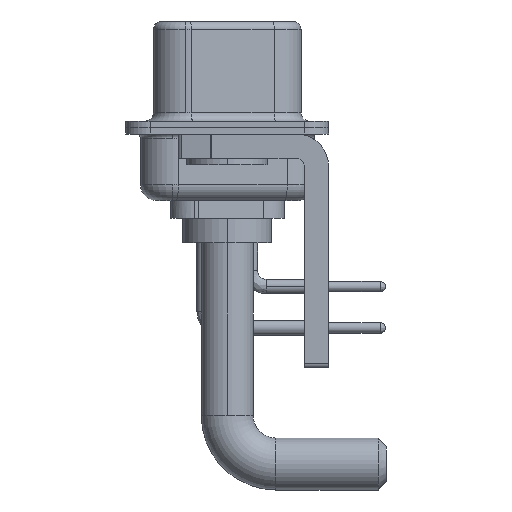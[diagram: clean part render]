
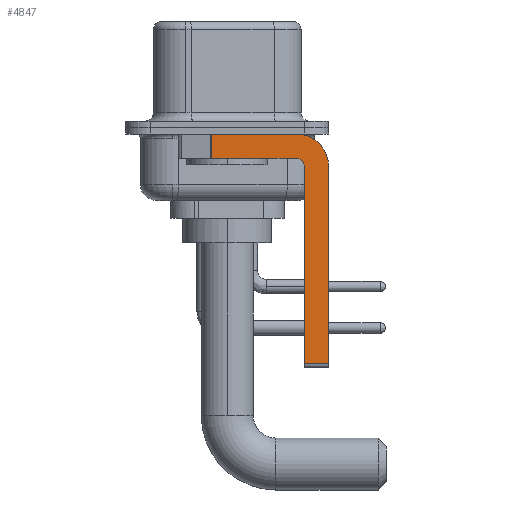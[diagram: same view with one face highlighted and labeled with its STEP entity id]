
A CAD part, left-side view. The second image highlights one B-rep face of the part: STEP entity #4847.
In plain terms, the highlighted planar face has unit normal (-1, 0, 0).
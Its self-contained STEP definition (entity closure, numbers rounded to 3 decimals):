
#95 = DIRECTION ( 'NONE',  ( 0., 0., 1. ) ) ;
#190 = DIRECTION ( 'NONE',  ( 0., 0., -1. ) ) ;
#220 = VECTOR ( 'NONE', #17806, 1000. ) ;
#597 = ORIENTED_EDGE ( 'NONE', *, *, #23594, .F. ) ;
#1214 = EDGE_CURVE ( 'NONE', #20308, #26542, #6845, .T. ) ;
#1604 = VECTOR ( 'NONE', #17730, 1000. ) ;
#2691 = EDGE_CURVE ( 'NONE', #11770, #5255, #26349, .T. ) ;
#4847 = ADVANCED_FACE ( 'NONE', ( #18382 ), #9376, .F. ) ;
#5215 = EDGE_CURVE ( 'NONE', #26542, #19874, #8018, .T. ) ;
#5255 = VERTEX_POINT ( 'NONE', #9340 ) ;
#6845 = CIRCLE ( 'NONE', #14374, 2. ) ;
#7545 = DIRECTION ( 'NONE',  ( -1., 0., 0. ) ) ;
#8018 = LINE ( 'NONE', #26253, #20402 ) ;
#8650 = ORIENTED_EDGE ( 'NONE', *, *, #5215, .F. ) ;
#8683 = DIRECTION ( 'NONE',  ( 1., 0., 0. ) ) ;
#8700 = CARTESIAN_POINT ( 'NONE',  ( -2.9, -6.25, -14.55 ) ) ;
#8713 = LINE ( 'NONE', #11353, #1604 ) ;
#9340 = CARTESIAN_POINT ( 'NONE',  ( -2.9, -4.25, -1.9 ) ) ;
#9376 = PLANE ( 'NONE',  #21688 ) ;
#9439 = DIRECTION ( 'NONE',  ( 0., 1., 0. ) ) ;
#9688 = ORIENTED_EDGE ( 'NONE', *, *, #2691, .F. ) ;
#10058 = CARTESIAN_POINT ( 'NONE',  ( -2.9, -6.25, -2.4 ) ) ;
#11004 = LINE ( 'NONE', #24619, #220 ) ;
#11353 = CARTESIAN_POINT ( 'NONE',  ( -2.9, 3., -0.4 ) ) ;
#11670 = DIRECTION ( 'NONE',  ( 0., 0., -1. ) ) ;
#11770 = VERTEX_POINT ( 'NONE', #20840 ) ;
#12205 = ORIENTED_EDGE ( 'NONE', *, *, #20046, .F. ) ;
#12798 = ORIENTED_EDGE ( 'NONE', *, *, #27041, .T. ) ;
#13275 = ORIENTED_EDGE ( 'NONE', *, *, #23875, .T. ) ;
#13927 = VERTEX_POINT ( 'NONE', #18630 ) ;
#14374 = AXIS2_PLACEMENT_3D ( 'NONE', #23363, #25442, #11670 ) ;
#14714 = CARTESIAN_POINT ( 'NONE',  ( -2.9, -4.25, -0.4 ) ) ;
#14962 = DIRECTION ( 'NONE',  ( 0., 0., -1. ) ) ;
#15171 = LINE ( 'NONE', #17241, #24288 ) ;
#15941 = CARTESIAN_POINT ( 'NONE',  ( -2.9, -4.25, -1.9 ) ) ;
#16062 = ORIENTED_EDGE ( 'NONE', *, *, #1214, .F. ) ;
#16559 = DIRECTION ( 'NONE',  ( 0., 0., 1. ) ) ;
#16741 = VECTOR ( 'NONE', #9439, 1000. ) ;
#17241 = CARTESIAN_POINT ( 'NONE',  ( -2.9, 0.978, -1.9 ) ) ;
#17318 = VERTEX_POINT ( 'NONE', #28801 ) ;
#17326 = AXIS2_PLACEMENT_3D ( 'NONE', #28012, #7545, #16559 ) ;
#17730 = DIRECTION ( 'NONE',  ( 0., -1., 0. ) ) ;
#17806 = DIRECTION ( 'NONE',  ( 0., -1., 0. ) ) ;
#18382 = FACE_OUTER_BOUND ( 'NONE', #19099, .T. ) ;
#18630 = CARTESIAN_POINT ( 'NONE',  ( -2.9, 0.978, -1.9 ) ) ;
#19099 = EDGE_LOOP ( 'NONE', ( #597, #13275, #19787, #9688, #12205, #12798, #8650, #16062 ) ) ;
#19787 = ORIENTED_EDGE ( 'NONE', *, *, #26929, .F. ) ;
#19874 = VERTEX_POINT ( 'NONE', #8700 ) ;
#20046 = EDGE_CURVE ( 'NONE', #21543, #11770, #22459, .T. ) ;
#20308 = VERTEX_POINT ( 'NONE', #14714 ) ;
#20402 = VECTOR ( 'NONE', #14962, 1000. ) ;
#20840 = CARTESIAN_POINT ( 'NONE',  ( -2.9, -4.75, -2.4 ) ) ;
#21248 = VECTOR ( 'NONE', #95, 1000. ) ;
#21543 = VERTEX_POINT ( 'NONE', #28985 ) ;
#21688 = AXIS2_PLACEMENT_3D ( 'NONE', #27444, #8683, #190 ) ;
#22459 = LINE ( 'NONE', #22609, #21248 ) ;
#22609 = CARTESIAN_POINT ( 'NONE',  ( -2.9, -4.75, -14.8 ) ) ;
#23363 = CARTESIAN_POINT ( 'NONE',  ( -2.9, -4.25, -2.4 ) ) ;
#23452 = LINE ( 'NONE', #15941, #16741 ) ;
#23594 = EDGE_CURVE ( 'NONE', #17318, #20308, #8713, .T. ) ;
#23875 = EDGE_CURVE ( 'NONE', #17318, #13927, #15171, .T. ) ;
#24288 = VECTOR ( 'NONE', #26318, 1000. ) ;
#24619 = CARTESIAN_POINT ( 'NONE',  ( -2.9, -4.25, -14.55 ) ) ;
#25442 = DIRECTION ( 'NONE',  ( 1., 0., 0. ) ) ;
#26253 = CARTESIAN_POINT ( 'NONE',  ( -2.9, -6.25, -2.4 ) ) ;
#26318 = DIRECTION ( 'NONE',  ( 0., 0., -1. ) ) ;
#26349 = CIRCLE ( 'NONE', #17326, 0.5 ) ;
#26542 = VERTEX_POINT ( 'NONE', #10058 ) ;
#26929 = EDGE_CURVE ( 'NONE', #5255, #13927, #23452, .T. ) ;
#27041 = EDGE_CURVE ( 'NONE', #21543, #19874, #11004, .T. ) ;
#27444 = CARTESIAN_POINT ( 'NONE',  ( -2.9, -4.25, -2.4 ) ) ;
#28012 = CARTESIAN_POINT ( 'NONE',  ( -2.9, -4.25, -2.4 ) ) ;
#28801 = CARTESIAN_POINT ( 'NONE',  ( -2.9, 0.978, -0.4 ) ) ;
#28985 = CARTESIAN_POINT ( 'NONE',  ( -2.9, -4.75, -14.55 ) ) ;
